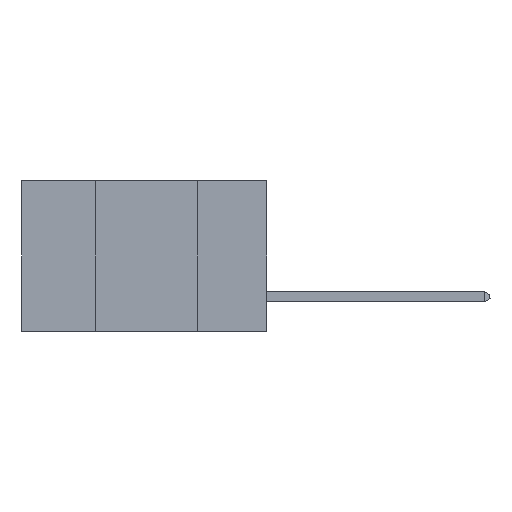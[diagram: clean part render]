
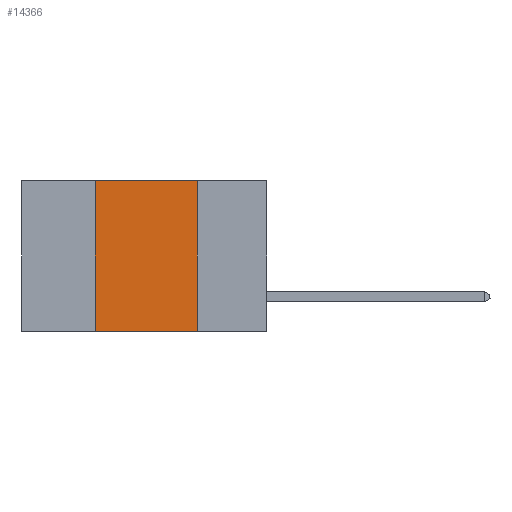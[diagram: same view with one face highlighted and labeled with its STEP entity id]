
A CAD part, left-side view. The second image highlights one B-rep face of the part: STEP entity #14366.
In plain terms, the highlighted planar face has unit normal (-1, 0, 0).
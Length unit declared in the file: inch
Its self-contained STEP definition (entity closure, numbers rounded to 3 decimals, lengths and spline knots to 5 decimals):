
#435 = VECTOR ( 'NONE', #14540, 39.37008 ) ;
#1525 = CARTESIAN_POINT ( 'NONE',  ( 0., 0.17, -0.37 ) ) ;
#2376 = DIRECTION ( 'NONE',  ( 0., -1., 0. ) ) ;
#3871 = VERTEX_POINT ( 'NONE', #1525 ) ;
#4086 = DIRECTION ( 'NONE',  ( 0., 0., -1. ) ) ;
#4829 = ORIENTED_EDGE ( 'NONE', *, *, #12764, .F. ) ;
#8620 = CARTESIAN_POINT ( 'NONE',  ( 0., 0.42, 0. ) ) ;
#12439 = ORIENTED_EDGE ( 'NONE', *, *, #35214, .F. ) ;
#12764 = EDGE_CURVE ( 'NONE', #14408, #21382, #28272, .T. ) ;
#14366 = ADVANCED_FACE ( 'NONE', ( #15902 ), #26325, .F. ) ;
#14408 = VERTEX_POINT ( 'NONE', #27306 ) ;
#14540 = DIRECTION ( 'NONE',  ( 0., 0., -1. ) ) ;
#15239 = EDGE_CURVE ( 'NONE', #41948, #3871, #21619, .T. ) ;
#15902 = FACE_OUTER_BOUND ( 'NONE', #43874, .T. ) ;
#19886 = ORIENTED_EDGE ( 'NONE', *, *, #15239, .T. ) ;
#21382 = VERTEX_POINT ( 'NONE', #23786 ) ;
#21619 = LINE ( 'NONE', #32018, #36366 ) ;
#23661 = DIRECTION ( 'NONE',  ( 0., 0., 1. ) ) ;
#23786 = CARTESIAN_POINT ( 'NONE',  ( 0., 0.17, 0. ) ) ;
#24343 = EDGE_CURVE ( 'NONE', #41948, #14408, #46734, .T. ) ;
#26325 = PLANE ( 'NONE',  #44751 ) ;
#26815 = CARTESIAN_POINT ( 'NONE',  ( 0., 0.6, 0. ) ) ;
#27306 = CARTESIAN_POINT ( 'NONE',  ( 0., 0.42, 0. ) ) ;
#28272 = LINE ( 'NONE', #33037, #47051 ) ;
#31522 = LINE ( 'NONE', #48420, #435 ) ;
#32018 = CARTESIAN_POINT ( 'NONE',  ( 0., 0.6, -0.37 ) ) ;
#32574 = DIRECTION ( 'NONE',  ( 0., -1., 0. ) ) ;
#33037 = CARTESIAN_POINT ( 'NONE',  ( 0., 0.6, 0. ) ) ;
#33324 = CARTESIAN_POINT ( 'NONE',  ( 0., 0.42, -0.37 ) ) ;
#34580 = DIRECTION ( 'NONE',  ( 1., 0., 0. ) ) ;
#35214 = EDGE_CURVE ( 'NONE', #21382, #3871, #31522, .T. ) ;
#36269 = VECTOR ( 'NONE', #23661, 39.37008 ) ;
#36366 = VECTOR ( 'NONE', #2376, 39.37008 ) ;
#38524 = ORIENTED_EDGE ( 'NONE', *, *, #24343, .F. ) ;
#41948 = VERTEX_POINT ( 'NONE', #33324 ) ;
#43874 = EDGE_LOOP ( 'NONE', ( #12439, #4829, #38524, #19886 ) ) ;
#44751 = AXIS2_PLACEMENT_3D ( 'NONE', #26815, #34580, #4086 ) ;
#46734 = LINE ( 'NONE', #8620, #36269 ) ;
#47051 = VECTOR ( 'NONE', #32574, 39.37008 ) ;
#48420 = CARTESIAN_POINT ( 'NONE',  ( 0., 0.17, 0. ) ) ;
